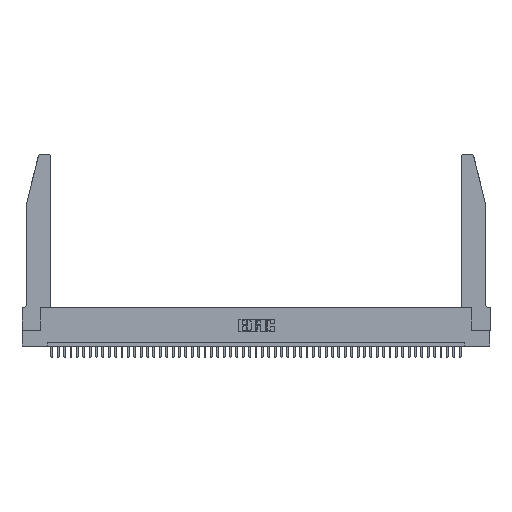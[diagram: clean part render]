
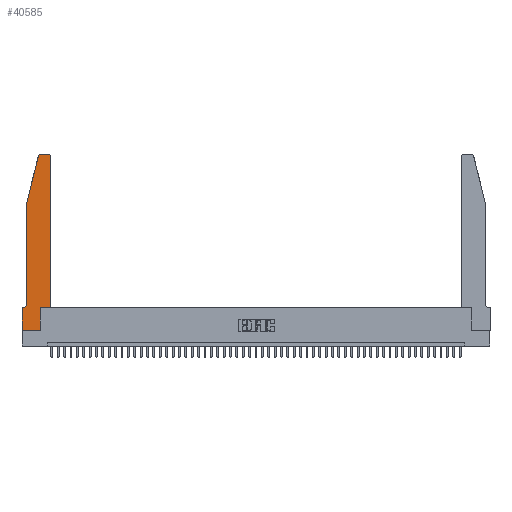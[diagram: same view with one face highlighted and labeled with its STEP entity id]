
A CAD part, top view. The second image highlights one B-rep face of the part: STEP entity #40585.
In plain terms, the highlighted planar face has unit normal (0, 0, 1).
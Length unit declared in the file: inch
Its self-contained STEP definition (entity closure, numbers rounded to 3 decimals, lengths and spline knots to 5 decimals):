
#9 = AXIS2_PLACEMENT_3D ( 'NONE', #45089, #1987, #29285 ) ;
#897 = EDGE_CURVE ( 'NONE', #13381, #23167, #49250, .T. ) ;
#1022 = CARTESIAN_POINT ( 'NONE',  ( 0., 0.35, 0.37 ) ) ;
#1324 = DIRECTION ( 'NONE',  ( -1., 0., 0. ) ) ;
#1987 = DIRECTION ( 'NONE',  ( 0., 0., 1. ) ) ;
#3267 = DIRECTION ( 'NONE',  ( 1., 0., 0. ) ) ;
#3468 = VECTOR ( 'NONE', #32538, 39.37008 ) ;
#4123 = DIRECTION ( 'NONE',  ( 0., 1., 0. ) ) ;
#4750 = VERTEX_POINT ( 'NONE', #1022 ) ;
#4940 = LINE ( 'NONE', #18733, #46622 ) ;
#5184 = CARTESIAN_POINT ( 'NONE',  ( 0., 0.35, 0.37 ) ) ;
#5546 = CARTESIAN_POINT ( 'NONE',  ( 0., 0., 0.37 ) ) ;
#5967 = EDGE_CURVE ( 'NONE', #25692, #13381, #34697, .T. ) ;
#7860 = CARTESIAN_POINT ( 'NONE',  ( 0.4505, 0.35, 0.37 ) ) ;
#8107 = ORIENTED_EDGE ( 'NONE', *, *, #49858, .T. ) ;
#8703 = DIRECTION ( 'NONE',  ( 0., -1., 0. ) ) ;
#8712 = AXIS2_PLACEMENT_3D ( 'NONE', #5184, #32683, #28756 ) ;
#8911 = PLANE ( 'NONE',  #8712 ) ;
#9026 = CARTESIAN_POINT ( 'NONE',  ( 0.0755, 2., 0.37 ) ) ;
#9694 = DIRECTION ( 'NONE',  ( 0., 1., 0. ) ) ;
#9698 = VERTEX_POINT ( 'NONE', #32582 ) ;
#9937 = ORIENTED_EDGE ( 'NONE', *, *, #32870, .T. ) ;
#10188 = VECTOR ( 'NONE', #28621, 39.37008 ) ;
#10217 = CARTESIAN_POINT ( 'NONE',  ( 0., 0., 0.37 ) ) ;
#10353 = VECTOR ( 'NONE', #8703, 39.37008 ) ;
#10631 = EDGE_CURVE ( 'NONE', #37138, #17108, #39029, .T. ) ;
#11970 = CARTESIAN_POINT ( 'NONE',  ( 0.0755, 0.42, 0.37 ) ) ;
#13381 = VERTEX_POINT ( 'NONE', #16968 ) ;
#16968 = CARTESIAN_POINT ( 'NONE',  ( 0.2865, 0., 0.37 ) ) ;
#17108 = VERTEX_POINT ( 'NONE', #42661 ) ;
#17113 = ORIENTED_EDGE ( 'NONE', *, *, #20520, .T. ) ;
#17648 = VERTEX_POINT ( 'NONE', #11970 ) ;
#18733 = CARTESIAN_POINT ( 'NONE',  ( 0.4505, 0.35, 0.37 ) ) ;
#19292 = EDGE_CURVE ( 'NONE', #23167, #24164, #4940, .T. ) ;
#20520 = EDGE_CURVE ( 'NONE', #38334, #37138, #47125, .T. ) ;
#21036 = CARTESIAN_POINT ( 'NONE',  ( 0.4205, 2.75, 0.37 ) ) ;
#21125 = ORIENTED_EDGE ( 'NONE', *, *, #26434, .T. ) ;
#21728 = CARTESIAN_POINT ( 'NONE',  ( 0.0055, 0.42, 0.37 ) ) ;
#23167 = VERTEX_POINT ( 'NONE', #44363 ) ;
#23977 = ORIENTED_EDGE ( 'NONE', *, *, #10631, .T. ) ;
#24164 = VERTEX_POINT ( 'NONE', #40020 ) ;
#24262 = CIRCLE ( 'NONE', #47354, 0.07 ) ;
#25692 = VERTEX_POINT ( 'NONE', #10217 ) ;
#25875 = DIRECTION ( 'NONE',  ( 0., 0., -1. ) ) ;
#26029 = CARTESIAN_POINT ( 'NONE',  ( 0.284, 2.75, 0.37 ) ) ;
#26135 = ORIENTED_EDGE ( 'NONE', *, *, #31141, .T. ) ;
#26434 = EDGE_CURVE ( 'NONE', #17648, #30337, #24262, .T. ) ;
#27588 = VERTEX_POINT ( 'NONE', #29848 ) ;
#27984 = DIRECTION ( 'NONE',  ( -0.239, -0.971, 0. ) ) ;
#28452 = CARTESIAN_POINT ( 'NONE',  ( 0.2605, 2.75, 0.37 ) ) ;
#28615 = LINE ( 'NONE', #43735, #3468 ) ;
#28621 = DIRECTION ( 'NONE',  ( 0., -1., 0. ) ) ;
#28756 = DIRECTION ( 'NONE',  ( 1., 0., 0. ) ) ;
#28818 = EDGE_CURVE ( 'NONE', #17108, #9698, #38769, .T. ) ;
#29285 = DIRECTION ( 'NONE',  ( 1., 0., 0. ) ) ;
#29848 = CARTESIAN_POINT ( 'NONE',  ( 0.4505, 2.72, 0.37 ) ) ;
#29922 = CARTESIAN_POINT ( 'NONE',  ( 0.0055, 0.35, 0.37 ) ) ;
#30337 = VERTEX_POINT ( 'NONE', #29922 ) ;
#31141 = EDGE_CURVE ( 'NONE', #30337, #4750, #28615, .T. ) ;
#31597 = ORIENTED_EDGE ( 'NONE', *, *, #897, .T. ) ;
#32210 = VECTOR ( 'NONE', #32550, 39.37008 ) ;
#32538 = DIRECTION ( 'NONE',  ( -1., 0., 0. ) ) ;
#32550 = DIRECTION ( 'NONE',  ( 1., 0., 0. ) ) ;
#32582 = CARTESIAN_POINT ( 'NONE',  ( 0.0755, 2., 0.37 ) ) ;
#32683 = DIRECTION ( 'NONE',  ( 0., 0., 1. ) ) ;
#32870 = EDGE_CURVE ( 'NONE', #24164, #27588, #36212, .T. ) ;
#33656 = VECTOR ( 'NONE', #1324, 39.37008 ) ;
#33992 = DIRECTION ( 'NONE',  ( 0., 0., 1. ) ) ;
#34319 = DIRECTION ( 'NONE',  ( 1., 0., 0. ) ) ;
#34697 = LINE ( 'NONE', #5546, #32210 ) ;
#34700 = EDGE_LOOP ( 'NONE', ( #17113, #23977, #38243, #8107, #21125, #26135, #44768, #40800, #31597, #39048, #9937, #37347 ) ) ;
#36212 = LINE ( 'NONE', #7860, #41766 ) ;
#36637 = EDGE_CURVE ( 'NONE', #27588, #38334, #46335, .T. ) ;
#37138 = VERTEX_POINT ( 'NONE', #26029 ) ;
#37347 = ORIENTED_EDGE ( 'NONE', *, *, #36637, .T. ) ;
#38243 = ORIENTED_EDGE ( 'NONE', *, *, #28818, .T. ) ;
#38334 = VERTEX_POINT ( 'NONE', #21036 ) ;
#38769 = LINE ( 'NONE', #43787, #50404 ) ;
#38877 = VECTOR ( 'NONE', #9694, 39.37008 ) ;
#39029 = CIRCLE ( 'NONE', #9, 0.03 ) ;
#39048 = ORIENTED_EDGE ( 'NONE', *, *, #19292, .T. ) ;
#39182 = LINE ( 'NONE', #9026, #10353 ) ;
#40020 = CARTESIAN_POINT ( 'NONE',  ( 0.4505, 0.35, 0.37 ) ) ;
#40507 = CARTESIAN_POINT ( 'NONE',  ( 0., 0., 0.37 ) ) ;
#40585 = ADVANCED_FACE ( 'NONE', ( #46644 ), #8911, .T. ) ;
#40800 = ORIENTED_EDGE ( 'NONE', *, *, #5967, .T. ) ;
#41766 = VECTOR ( 'NONE', #4123, 39.37008 ) ;
#42661 = CARTESIAN_POINT ( 'NONE',  ( 0.25487, 2.72718, 0.37 ) ) ;
#42712 = LINE ( 'NONE', #40507, #10188 ) ;
#43735 = CARTESIAN_POINT ( 'NONE',  ( 0.0755, 0.35, 0.37 ) ) ;
#43787 = CARTESIAN_POINT ( 'NONE',  ( 0.0755, 2., 0.37 ) ) ;
#43806 = EDGE_CURVE ( 'NONE', #4750, #25692, #42712, .T. ) ;
#44363 = CARTESIAN_POINT ( 'NONE',  ( 0.2865, 0.35, 0.37 ) ) ;
#44768 = ORIENTED_EDGE ( 'NONE', *, *, #43806, .T. ) ;
#45017 = CARTESIAN_POINT ( 'NONE',  ( 0.2865, 0.35, 0.37 ) ) ;
#45089 = CARTESIAN_POINT ( 'NONE',  ( 0.284, 2.72, 0.37 ) ) ;
#45442 = DIRECTION ( 'NONE',  ( -1., 0., 0. ) ) ;
#46335 = CIRCLE ( 'NONE', #47362, 0.03 ) ;
#46622 = VECTOR ( 'NONE', #3267, 39.37008 ) ;
#46644 = FACE_OUTER_BOUND ( 'NONE', #34700, .T. ) ;
#47125 = LINE ( 'NONE', #28452, #33656 ) ;
#47354 = AXIS2_PLACEMENT_3D ( 'NONE', #21728, #25875, #45442 ) ;
#47362 = AXIS2_PLACEMENT_3D ( 'NONE', #49926, #33992, #34319 ) ;
#49250 = LINE ( 'NONE', #45017, #38877 ) ;
#49858 = EDGE_CURVE ( 'NONE', #9698, #17648, #39182, .T. ) ;
#49926 = CARTESIAN_POINT ( 'NONE',  ( 0.4205, 2.72, 0.37 ) ) ;
#50404 = VECTOR ( 'NONE', #27984, 39.37008 ) ;
